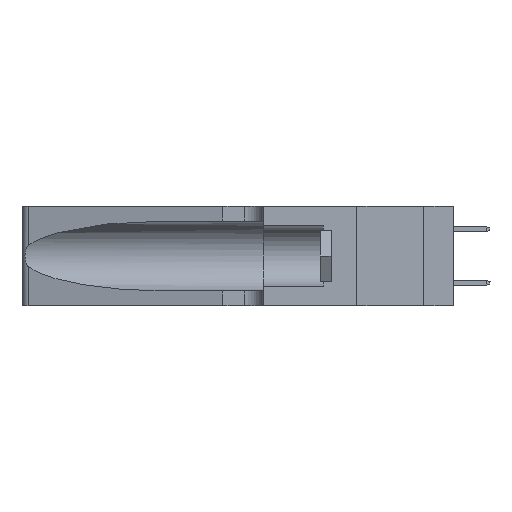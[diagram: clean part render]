
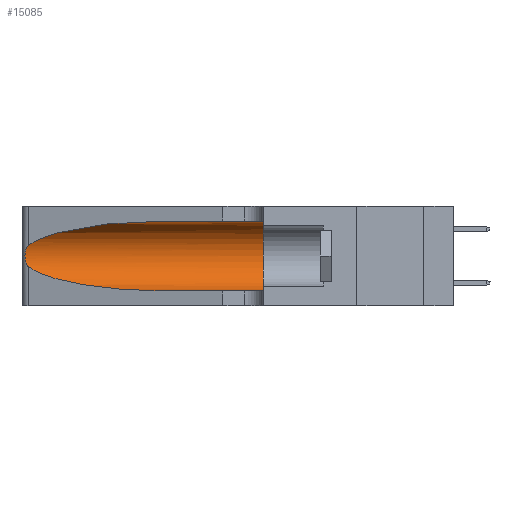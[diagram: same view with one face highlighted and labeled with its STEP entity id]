
A CAD part, left-side view. The second image highlights one B-rep face of the part: STEP entity #15085.
In plain terms, the highlighted cylindrical face has radius 3.308 mm (diameter 6.617 mm), a partial arc.
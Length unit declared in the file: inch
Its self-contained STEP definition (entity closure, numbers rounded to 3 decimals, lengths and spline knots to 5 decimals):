
#198 = CARTESIAN_POINT ( 'NONE',  ( 0.25555, 1.22993, 0.14849 ) ) ;
#387 = AXIS2_PLACEMENT_3D ( 'NONE', #7664, #12582, #20843 ) ;
#558 = VERTEX_POINT ( 'NONE', #4727 ) ;
#706 = CARTESIAN_POINT ( 'NONE',  ( 0.2373, 1.15595, 0.08982 ) ) ;
#969 = ORIENTED_EDGE ( 'NONE', *, *, #19715, .T. ) ;
#988 = CARTESIAN_POINT ( 'NONE',  ( 0.1305, 0.35, 0.31525 ) ) ;
#1067 = CARTESIAN_POINT ( 'NONE',  ( 0.25487, 1.22718, 0.22369 ) ) ;
#1842 = CARTESIAN_POINT ( 'NONE',  ( 0.26017, 1.23833, 0.17102 ) ) ;
#2290 = CARTESIAN_POINT ( 'NONE',  ( 0.25487, 1.22718, 0.22369 ) ) ;
#2419 = CARTESIAN_POINT ( 'NONE',  ( 0.1305, 0.72297, 0.05475 ) ) ;
#3090 = VERTEX_POINT ( 'NONE', #12978 ) ;
#3158 = EDGE_CURVE ( 'NONE', #20617, #3090, #18484, .T. ) ;
#3649 = CARTESIAN_POINT ( 'NONE',  ( 0.25487, 1.22718, 0.22369 ) ) ;
#3802 = CARTESIAN_POINT ( 'NONE',  ( 0.25789, 1.23486, 0.15765 ) ) ;
#4727 = CARTESIAN_POINT ( 'NONE',  ( 0.1305, 0.72297, 0.31525 ) ) ;
#5123 = CARTESIAN_POINT ( 'NONE',  ( 0.25787, 1.23484, 0.2124 ) ) ;
#5169 =( BOUNDED_CURVE ( )  B_SPLINE_CURVE ( 3, ( #20801, #706, #10786, #7194 ),
 .UNSPECIFIED., .F., .T. ) 
 B_SPLINE_CURVE_WITH_KNOTS ( ( 4, 4 ),
 ( 3.44316, 4.71239 ),
 .UNSPECIFIED. ) 
 CURVE ( )  GEOMETRIC_REPRESENTATION_ITEM ( )  RATIONAL_B_SPLINE_CURVE ( ( 1., 0.87, 0.87, 1. ) ) 
 REPRESENTATION_ITEM ( '' )  );
#5201 = CARTESIAN_POINT ( 'NONE',  ( 0.2373, 1.15595, 0.28018 ) ) ;
#5249 = ORIENTED_EDGE ( 'NONE', *, *, #18345, .T. ) ;
#5308 = CARTESIAN_POINT ( 'NONE',  ( 0.18966, 0.96281, 0.31525 ) ) ;
#5460 = CARTESIAN_POINT ( 'NONE',  ( 0.25856, 1.23593, 0.16098 ) ) ;
#5874 = VECTOR ( 'NONE', #9763, 39.37008 ) ;
#5994 = DIRECTION ( 'NONE',  ( 0., 1., 0. ) ) ;
#6998 = CARTESIAN_POINT ( 'NONE',  ( 0.26075, 1.23896, 0.178 ) ) ;
#7106 = CARTESIAN_POINT ( 'NONE',  ( 0.25854, 1.2359, 0.20912 ) ) ;
#7128 = EDGE_CURVE ( 'NONE', #558, #15081, #9516, .T. ) ;
#7194 = CARTESIAN_POINT ( 'NONE',  ( 0.1305, 0.72297, 0.05475 ) ) ;
#7227 = CARTESIAN_POINT ( 'NONE',  ( 0.25639, 1.23184, 0.21858 ) ) ;
#7652 = CARTESIAN_POINT ( 'NONE',  ( 0.1305, 0.35, 0.185 ) ) ;
#7664 = CARTESIAN_POINT ( 'NONE',  ( 0.1305, 1.61858, 0.185 ) ) ;
#7738 = VERTEX_POINT ( 'NONE', #9993 ) ;
#8354 = VECTOR ( 'NONE', #16814, 39.37008 ) ;
#8864 = CARTESIAN_POINT ( 'NONE',  ( 0.25487, 1.22718, 0.14631 ) ) ;
#9516 =( BOUNDED_CURVE ( )  B_SPLINE_CURVE ( 3, ( #14637, #5308, #5201, #3649 ),
 .UNSPECIFIED., .F., .T. ) 
 B_SPLINE_CURVE_WITH_KNOTS ( ( 4, 4 ),
 ( 1.5708, 2.84003 ),
 .UNSPECIFIED. ) 
 CURVE ( )  GEOMETRIC_REPRESENTATION_ITEM ( )  RATIONAL_B_SPLINE_CURVE ( ( 1., 0.87, 0.87, 1. ) ) 
 REPRESENTATION_ITEM ( '' )  );
#9763 = DIRECTION ( 'NONE',  ( 0., -1., 0. ) ) ;
#9993 = CARTESIAN_POINT ( 'NONE',  ( 0.25487, 1.22718, 0.14631 ) ) ;
#10390 = EDGE_CURVE ( 'NONE', #558, #17584, #21312, .T. ) ;
#10725 = CYLINDRICAL_SURFACE ( 'NONE', #387, 0.13025 ) ;
#10786 = CARTESIAN_POINT ( 'NONE',  ( 0.18966, 0.96281, 0.05475 ) ) ;
#11303 = EDGE_CURVE ( 'NONE', #17584, #3090, #20232, .T. ) ;
#11388 = B_SPLINE_CURVE_WITH_KNOTS ( 'NONE', 3,
 ( #2290, #18970, #7227, #5123, #7106, #18861, #15106, #6998, #1842, #5460, #3802, #20281, #198, #8864 ),
 .UNSPECIFIED., .F., .F.,
 ( 4, 2, 2, 2, 2, 2, 4 ),
 ( 0., 0.00027, 0.00053, 0.00107, 0.0016, 0.00187, 0.00214 ),
 .UNSPECIFIED. ) ;
#12582 = DIRECTION ( 'NONE',  ( 0., -1., 0. ) ) ;
#12626 = EDGE_LOOP ( 'NONE', ( #15845, #969, #5249, #18640, #16582, #13689 ) ) ;
#12978 = CARTESIAN_POINT ( 'NONE',  ( 0.1305, 0.35, 0.05475 ) ) ;
#13393 = CARTESIAN_POINT ( 'NONE',  ( 0.1305, 1.61858, 0.05475 ) ) ;
#13689 = ORIENTED_EDGE ( 'NONE', *, *, #10390, .F. ) ;
#14320 = DIRECTION ( 'NONE',  ( 0., 0., 1. ) ) ;
#14637 = CARTESIAN_POINT ( 'NONE',  ( 0.1305, 0.72297, 0.31525 ) ) ;
#15081 = VERTEX_POINT ( 'NONE', #1067 ) ;
#15085 = ADVANCED_FACE ( 'NONE', ( #15780 ), #10725, .F. ) ;
#15106 = CARTESIAN_POINT ( 'NONE',  ( 0.26075, 1.23896, 0.19203 ) ) ;
#15780 = FACE_OUTER_BOUND ( 'NONE', #12626, .T. ) ;
#15845 = ORIENTED_EDGE ( 'NONE', *, *, #7128, .T. ) ;
#16582 = ORIENTED_EDGE ( 'NONE', *, *, #11303, .F. ) ;
#16814 = DIRECTION ( 'NONE',  ( 0., -1., 0. ) ) ;
#17584 = VERTEX_POINT ( 'NONE', #988 ) ;
#18345 = EDGE_CURVE ( 'NONE', #7738, #20617, #5169, .T. ) ;
#18484 = LINE ( 'NONE', #13393, #8354 ) ;
#18491 = AXIS2_PLACEMENT_3D ( 'NONE', #7652, #5994, #14320 ) ;
#18640 = ORIENTED_EDGE ( 'NONE', *, *, #3158, .T. ) ;
#18861 = CARTESIAN_POINT ( 'NONE',  ( 0.26018, 1.23835, 0.19895 ) ) ;
#18970 = CARTESIAN_POINT ( 'NONE',  ( 0.25555, 1.22994, 0.2215 ) ) ;
#19715 = EDGE_CURVE ( 'NONE', #15081, #7738, #11388, .T. ) ;
#20232 = CIRCLE ( 'NONE', #18491, 0.13025 ) ;
#20281 = CARTESIAN_POINT ( 'NONE',  ( 0.25639, 1.23186, 0.15144 ) ) ;
#20617 = VERTEX_POINT ( 'NONE', #2419 ) ;
#20801 = CARTESIAN_POINT ( 'NONE',  ( 0.25487, 1.22718, 0.14631 ) ) ;
#20843 = DIRECTION ( 'NONE',  ( 0., 0., -1. ) ) ;
#21312 = LINE ( 'NONE', #21533, #5874 ) ;
#21533 = CARTESIAN_POINT ( 'NONE',  ( 0.1305, 1.61858, 0.31525 ) ) ;
